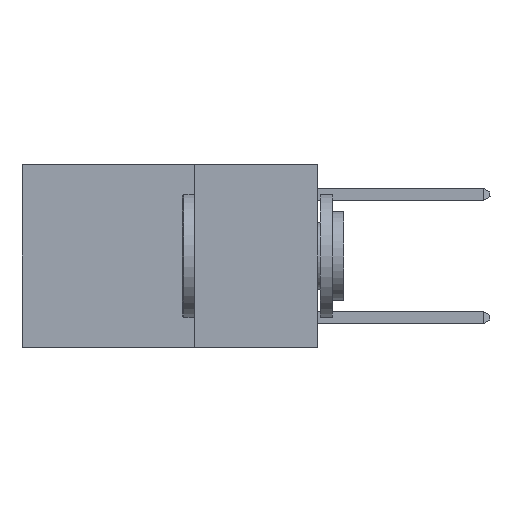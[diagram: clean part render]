
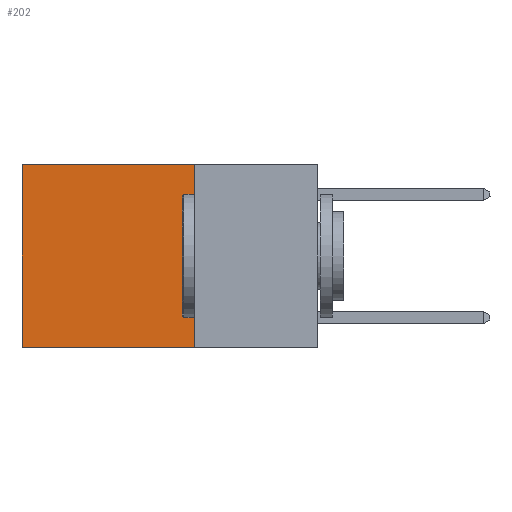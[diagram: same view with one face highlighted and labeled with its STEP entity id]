
A CAD part, left-side view. The second image highlights one B-rep face of the part: STEP entity #202.
In plain terms, the highlighted planar face has unit normal (-1, 0, 0).
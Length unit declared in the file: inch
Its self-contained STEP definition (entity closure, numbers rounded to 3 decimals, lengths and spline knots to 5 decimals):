
#200 = FACE_OUTER_BOUND ( 'NONE', #10593, .T. ) ;
#202 = ADVANCED_FACE ( 'NONE', ( #200 ), #28875, .F. ) ;
#1778 = LINE ( 'NONE', #23377, #18701 ) ;
#3804 = CARTESIAN_POINT ( 'NONE',  ( 0.2625, 0.6, -0.37 ) ) ;
#4815 = ORIENTED_EDGE ( 'NONE', *, *, #18244, .T. ) ;
#4959 = DIRECTION ( 'NONE',  ( 0., 0., -1. ) ) ;
#5803 = CARTESIAN_POINT ( 'NONE',  ( 0.2625, 0.25, -0.37 ) ) ;
#5819 = VERTEX_POINT ( 'NONE', #25133 ) ;
#7116 = CARTESIAN_POINT ( 'NONE',  ( 0.2625, 0.25, 0. ) ) ;
#7711 = LINE ( 'NONE', #26941, #22511 ) ;
#9488 = EDGE_CURVE ( 'NONE', #5819, #26128, #19298, .T. ) ;
#10400 = DIRECTION ( 'NONE',  ( 0., 1., 0. ) ) ;
#10593 = EDGE_LOOP ( 'NONE', ( #13241, #22911, #13160, #4815 ) ) ;
#11369 = VECTOR ( 'NONE', #10400, 39.37008 ) ;
#12770 = LINE ( 'NONE', #18116, #11369 ) ;
#12776 = VERTEX_POINT ( 'NONE', #21777 ) ;
#13160 = ORIENTED_EDGE ( 'NONE', *, *, #24570, .F. ) ;
#13241 = ORIENTED_EDGE ( 'NONE', *, *, #9488, .T. ) ;
#16789 = EDGE_CURVE ( 'NONE', #28182, #26128, #12770, .T. ) ;
#17190 = DIRECTION ( 'NONE',  ( 0., 0., -1. ) ) ;
#18116 = CARTESIAN_POINT ( 'NONE',  ( 0.2625, 0.25, -0.37 ) ) ;
#18244 = EDGE_CURVE ( 'NONE', #12776, #5819, #7711, .T. ) ;
#18701 = VECTOR ( 'NONE', #28264, 39.37008 ) ;
#18964 = CARTESIAN_POINT ( 'NONE',  ( 0.2625, 0.6, 0. ) ) ;
#19298 = LINE ( 'NONE', #18964, #29494 ) ;
#19527 = DIRECTION ( 'NONE',  ( 0., 1., 0. ) ) ;
#21777 = CARTESIAN_POINT ( 'NONE',  ( 0.2625, 0.25, 0. ) ) ;
#22511 = VECTOR ( 'NONE', #19527, 39.37008 ) ;
#22911 = ORIENTED_EDGE ( 'NONE', *, *, #16789, .F. ) ;
#23377 = CARTESIAN_POINT ( 'NONE',  ( 0.2625, 0.25, 0. ) ) ;
#24146 = DIRECTION ( 'NONE',  ( 1., 0., 0. ) ) ;
#24570 = EDGE_CURVE ( 'NONE', #12776, #28182, #1778, .T. ) ;
#25133 = CARTESIAN_POINT ( 'NONE',  ( 0.2625, 0.6, 0. ) ) ;
#26128 = VERTEX_POINT ( 'NONE', #3804 ) ;
#26941 = CARTESIAN_POINT ( 'NONE',  ( 0.2625, 0.25, 0. ) ) ;
#28182 = VERTEX_POINT ( 'NONE', #5803 ) ;
#28264 = DIRECTION ( 'NONE',  ( 0., 0., -1. ) ) ;
#28875 = PLANE ( 'NONE',  #28876 ) ;
#28876 = AXIS2_PLACEMENT_3D ( 'NONE', #7116, #24146, #17190 ) ;
#29494 = VECTOR ( 'NONE', #4959, 39.37008 ) ;
